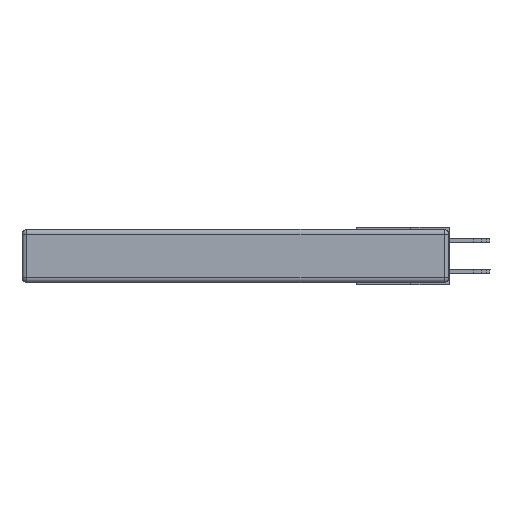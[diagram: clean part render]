
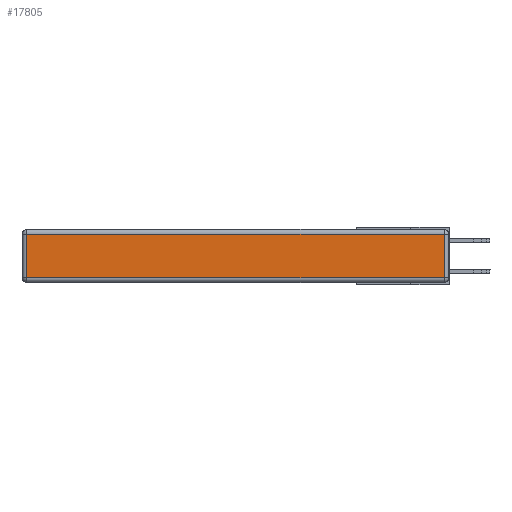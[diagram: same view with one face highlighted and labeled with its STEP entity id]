
A CAD part, left-side view. The second image highlights one B-rep face of the part: STEP entity #17805.
In plain terms, the highlighted planar face has unit normal (-1, 0, 0).
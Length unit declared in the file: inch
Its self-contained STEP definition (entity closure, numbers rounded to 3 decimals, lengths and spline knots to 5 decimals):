
#255 = LINE ( 'NONE', #20651, #22736 ) ;
#879 = CARTESIAN_POINT ( 'NONE',  ( 0., 2.72, -0.313 ) ) ;
#1478 = ORIENTED_EDGE ( 'NONE', *, *, #14827, .T. ) ;
#2171 = VERTEX_POINT ( 'NONE', #10981 ) ;
#2322 = ORIENTED_EDGE ( 'NONE', *, *, #12950, .T. ) ;
#2506 = ORIENTED_EDGE ( 'NONE', *, *, #24113, .T. ) ;
#2968 = DIRECTION ( 'NONE',  ( 0., 0., -1. ) ) ;
#3054 = VECTOR ( 'NONE', #21251, 39.37008 ) ;
#3375 = LINE ( 'NONE', #25444, #3054 ) ;
#4475 = VERTEX_POINT ( 'NONE', #18896 ) ;
#7027 = LINE ( 'NONE', #12545, #18891 ) ;
#9042 = DIRECTION ( 'NONE',  ( 0., 0., 1. ) ) ;
#9545 = FACE_OUTER_BOUND ( 'NONE', #26462, .T. ) ;
#10403 = DIRECTION ( 'NONE',  ( 0., 1., 0. ) ) ;
#10981 = CARTESIAN_POINT ( 'NONE',  ( 0., 0.03, -0.313 ) ) ;
#11257 = VECTOR ( 'NONE', #2968, 39.37008 ) ;
#12545 = CARTESIAN_POINT ( 'NONE',  ( 0., 2.75, -0.03 ) ) ;
#12950 = EDGE_CURVE ( 'NONE', #22612, #15113, #22552, .T. ) ;
#14815 = AXIS2_PLACEMENT_3D ( 'NONE', #17417, #22120, #9042 ) ;
#14827 = EDGE_CURVE ( 'NONE', #4475, #22612, #7027, .T. ) ;
#15113 = VERTEX_POINT ( 'NONE', #879 ) ;
#17417 = CARTESIAN_POINT ( 'NONE',  ( 0., 0., -0.343 ) ) ;
#17805 = ADVANCED_FACE ( 'NONE', ( #9545 ), #22009, .T. ) ;
#18891 = VECTOR ( 'NONE', #10403, 39.37008 ) ;
#18896 = CARTESIAN_POINT ( 'NONE',  ( 0., 0.03, -0.03 ) ) ;
#20651 = CARTESIAN_POINT ( 'NONE',  ( 0., 0., -0.313 ) ) ;
#20690 = EDGE_CURVE ( 'NONE', #15113, #2171, #255, .T. ) ;
#21251 = DIRECTION ( 'NONE',  ( 0., 0., 1. ) ) ;
#22009 = PLANE ( 'NONE',  #14815 ) ;
#22120 = DIRECTION ( 'NONE',  ( -1., 0., 0. ) ) ;
#22470 = CARTESIAN_POINT ( 'NONE',  ( 0., 2.72, -0.343 ) ) ;
#22552 = LINE ( 'NONE', #22470, #11257 ) ;
#22612 = VERTEX_POINT ( 'NONE', #23747 ) ;
#22736 = VECTOR ( 'NONE', #22868, 39.37008 ) ;
#22868 = DIRECTION ( 'NONE',  ( 0., -1., 0. ) ) ;
#23747 = CARTESIAN_POINT ( 'NONE',  ( 0., 2.72, -0.03 ) ) ;
#24113 = EDGE_CURVE ( 'NONE', #2171, #4475, #3375, .T. ) ;
#25444 = CARTESIAN_POINT ( 'NONE',  ( 0., 0.03, -0.343 ) ) ;
#26462 = EDGE_LOOP ( 'NONE', ( #26827, #2506, #1478, #2322 ) ) ;
#26827 = ORIENTED_EDGE ( 'NONE', *, *, #20690, .T. ) ;
